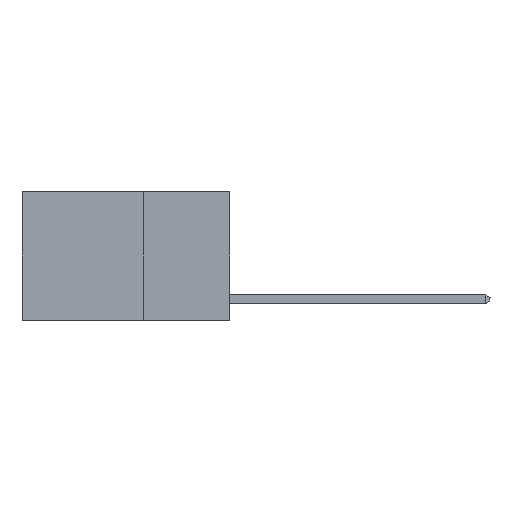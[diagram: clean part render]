
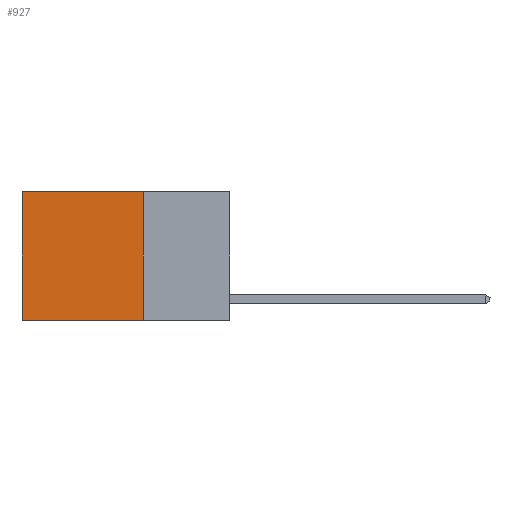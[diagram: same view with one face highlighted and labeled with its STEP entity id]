
A CAD part, left-side view. The second image highlights one B-rep face of the part: STEP entity #927.
In plain terms, the highlighted planar face has unit normal (-1, 0, 0).
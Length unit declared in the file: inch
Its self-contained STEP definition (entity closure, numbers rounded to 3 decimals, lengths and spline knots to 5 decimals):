
#163 = VECTOR ( 'NONE', #17355, 39.37008 ) ;
#512 = EDGE_CURVE ( 'NONE', #8686, #10867, #7645, .T. ) ;
#927 = ADVANCED_FACE ( 'NONE', ( #16965 ), #11840, .F. ) ;
#1310 = CARTESIAN_POINT ( 'NONE',  ( 0.2625, 0.6, 0. ) ) ;
#2104 = ORIENTED_EDGE ( 'NONE', *, *, #4427, .T. ) ;
#2705 = LINE ( 'NONE', #6032, #163 ) ;
#4012 = EDGE_CURVE ( 'NONE', #10867, #19607, #8254, .T. ) ;
#4315 = ORIENTED_EDGE ( 'NONE', *, *, #4012, .F. ) ;
#4427 = EDGE_CURVE ( 'NONE', #23195, #19607, #21214, .T. ) ;
#4446 = CARTESIAN_POINT ( 'NONE',  ( 0.2625, 0.25, -0.37 ) ) ;
#5353 = VECTOR ( 'NONE', #19502, 39.37008 ) ;
#6032 = CARTESIAN_POINT ( 'NONE',  ( 0.2625, 0.25, 0. ) ) ;
#6984 = CARTESIAN_POINT ( 'NONE',  ( 0.2625, 0.6, -0.37 ) ) ;
#7529 = CARTESIAN_POINT ( 'NONE',  ( 0.2625, 0.6, 0. ) ) ;
#7645 = LINE ( 'NONE', #13196, #17798 ) ;
#8254 = LINE ( 'NONE', #4446, #13823 ) ;
#8686 = VERTEX_POINT ( 'NONE', #11789 ) ;
#9559 = DIRECTION ( 'NONE',  ( 0., 0., -1. ) ) ;
#10867 = VERTEX_POINT ( 'NONE', #21112 ) ;
#11789 = CARTESIAN_POINT ( 'NONE',  ( 0.2625, 0.25, 0. ) ) ;
#11840 = PLANE ( 'NONE',  #14034 ) ;
#13196 = CARTESIAN_POINT ( 'NONE',  ( 0.2625, 0.25, 0. ) ) ;
#13823 = VECTOR ( 'NONE', #19319, 39.37008 ) ;
#14034 = AXIS2_PLACEMENT_3D ( 'NONE', #21114, #19290, #9559 ) ;
#16904 = DIRECTION ( 'NONE',  ( 0., 0., -1. ) ) ;
#16965 = FACE_OUTER_BOUND ( 'NONE', #19872, .T. ) ;
#17032 = ORIENTED_EDGE ( 'NONE', *, *, #18523, .T. ) ;
#17355 = DIRECTION ( 'NONE',  ( 0., 1., 0. ) ) ;
#17798 = VECTOR ( 'NONE', #16904, 39.37008 ) ;
#18523 = EDGE_CURVE ( 'NONE', #8686, #23195, #2705, .T. ) ;
#19290 = DIRECTION ( 'NONE',  ( 1., 0., 0. ) ) ;
#19319 = DIRECTION ( 'NONE',  ( 0., 1., 0. ) ) ;
#19502 = DIRECTION ( 'NONE',  ( 0., 0., -1. ) ) ;
#19607 = VERTEX_POINT ( 'NONE', #6984 ) ;
#19872 = EDGE_LOOP ( 'NONE', ( #2104, #4315, #22324, #17032 ) ) ;
#21112 = CARTESIAN_POINT ( 'NONE',  ( 0.2625, 0.25, -0.37 ) ) ;
#21114 = CARTESIAN_POINT ( 'NONE',  ( 0.2625, 0.25, 0. ) ) ;
#21214 = LINE ( 'NONE', #1310, #5353 ) ;
#22324 = ORIENTED_EDGE ( 'NONE', *, *, #512, .F. ) ;
#23195 = VERTEX_POINT ( 'NONE', #7529 ) ;
